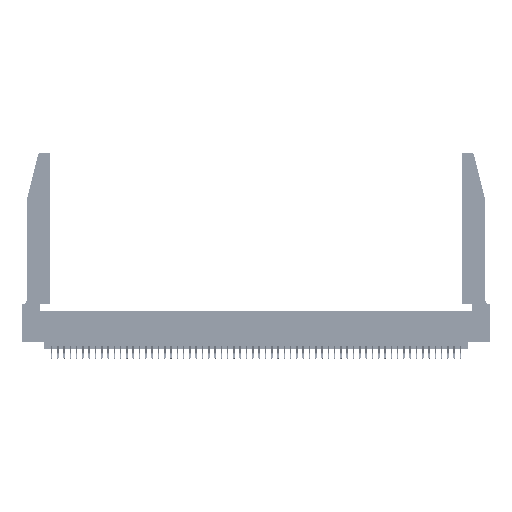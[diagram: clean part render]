
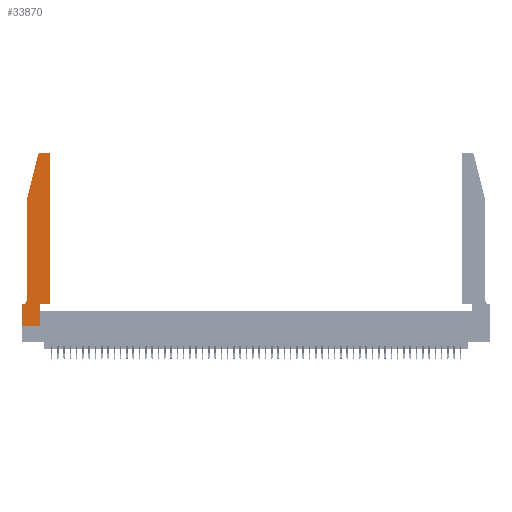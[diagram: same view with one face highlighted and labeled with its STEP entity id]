
A CAD part, top view. The second image highlights one B-rep face of the part: STEP entity #33870.
In plain terms, the highlighted planar face has unit normal (0, 0, 1).
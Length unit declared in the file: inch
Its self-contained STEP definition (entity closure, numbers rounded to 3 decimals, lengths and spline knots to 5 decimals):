
#320 = CARTESIAN_POINT ( 'NONE',  ( 0.0055, 0.35, 0.37 ) ) ;
#573 = LINE ( 'NONE', #35285, #25975 ) ;
#714 = LINE ( 'NONE', #33054, #20214 ) ;
#1095 = DIRECTION ( 'NONE',  ( 1., 0., 0. ) ) ;
#1208 = DIRECTION ( 'NONE',  ( 1., 0., 0. ) ) ;
#1482 = VECTOR ( 'NONE', #1095, 39.37008 ) ;
#1571 = CARTESIAN_POINT ( 'NONE',  ( 0.4205, 2.75, 0.37 ) ) ;
#1722 = VERTEX_POINT ( 'NONE', #13991 ) ;
#2215 = CARTESIAN_POINT ( 'NONE',  ( 0.4505, 2.72, 0.37 ) ) ;
#2318 = CARTESIAN_POINT ( 'NONE',  ( 0.25487, 2.72718, 0.37 ) ) ;
#3125 = CARTESIAN_POINT ( 'NONE',  ( 0.284, 2.75, 0.37 ) ) ;
#3454 = DIRECTION ( 'NONE',  ( -1., 0., 0. ) ) ;
#3720 = DIRECTION ( 'NONE',  ( -1., 0., 0. ) ) ;
#4032 = EDGE_CURVE ( 'NONE', #37979, #1722, #18860, .T. ) ;
#5062 = LINE ( 'NONE', #25738, #34886 ) ;
#6139 = CIRCLE ( 'NONE', #44516, 0.07 ) ;
#6187 = DIRECTION ( 'NONE',  ( 1., 0., 0. ) ) ;
#6192 = VECTOR ( 'NONE', #19793, 39.37008 ) ;
#6794 = FACE_OUTER_BOUND ( 'NONE', #23313, .T. ) ;
#6897 = ORIENTED_EDGE ( 'NONE', *, *, #30292, .T. ) ;
#7027 = ORIENTED_EDGE ( 'NONE', *, *, #11025, .T. ) ;
#8003 = CARTESIAN_POINT ( 'NONE',  ( 0.0055, 0.42, 0.37 ) ) ;
#8296 = DIRECTION ( 'NONE',  ( 1., 0., 0. ) ) ;
#9598 = CARTESIAN_POINT ( 'NONE',  ( 0.284, 2.72, 0.37 ) ) ;
#9760 = ORIENTED_EDGE ( 'NONE', *, *, #29949, .T. ) ;
#9822 = ORIENTED_EDGE ( 'NONE', *, *, #43814, .T. ) ;
#10663 = DIRECTION ( 'NONE',  ( -0.239, -0.971, 0. ) ) ;
#11025 = EDGE_CURVE ( 'NONE', #13094, #11939, #714, .T. ) ;
#11257 = DIRECTION ( 'NONE',  ( 0., -1., 0. ) ) ;
#11314 = LINE ( 'NONE', #20490, #43032 ) ;
#11939 = VERTEX_POINT ( 'NONE', #3125 ) ;
#12610 = CARTESIAN_POINT ( 'NONE',  ( 0.0755, 2., 0.37 ) ) ;
#13094 = VERTEX_POINT ( 'NONE', #1571 ) ;
#13742 = DIRECTION ( 'NONE',  ( 0., 0., 1. ) ) ;
#13981 = DIRECTION ( 'NONE',  ( 0., 0., 1. ) ) ;
#13991 = CARTESIAN_POINT ( 'NONE',  ( 0.4505, 0.35, 0.37 ) ) ;
#15262 = CARTESIAN_POINT ( 'NONE',  ( 0., 0., 0.37 ) ) ;
#15283 = CARTESIAN_POINT ( 'NONE',  ( 0.0755, 2., 0.37 ) ) ;
#16522 = DIRECTION ( 'NONE',  ( 0., 0., -1. ) ) ;
#16576 = VERTEX_POINT ( 'NONE', #320 ) ;
#18341 = PLANE ( 'NONE',  #24719 ) ;
#18860 = LINE ( 'NONE', #29109, #21410 ) ;
#19793 = DIRECTION ( 'NONE',  ( 0., -1., 0. ) ) ;
#19970 = DIRECTION ( 'NONE',  ( 0., 1., 0. ) ) ;
#20214 = VECTOR ( 'NONE', #3720, 39.37008 ) ;
#20245 = DIRECTION ( 'NONE',  ( 0., 0., 1. ) ) ;
#20411 = AXIS2_PLACEMENT_3D ( 'NONE', #9598, #13742, #1208 ) ;
#20490 = CARTESIAN_POINT ( 'NONE',  ( 0.2865, 0.35, 0.37 ) ) ;
#21410 = VECTOR ( 'NONE', #50491, 39.37008 ) ;
#21869 = EDGE_CURVE ( 'NONE', #35267, #13094, #24520, .T. ) ;
#22278 = LINE ( 'NONE', #46572, #1482 ) ;
#22293 = DIRECTION ( 'NONE',  ( 0., 1., 0. ) ) ;
#22319 = CARTESIAN_POINT ( 'NONE',  ( 0., 0.35, 0.37 ) ) ;
#22506 = VECTOR ( 'NONE', #49002, 39.37008 ) ;
#23307 = CARTESIAN_POINT ( 'NONE',  ( 0.0755, 0.35, 0.37 ) ) ;
#23313 = EDGE_LOOP ( 'NONE', ( #7027, #6897, #34327, #27683, #42469, #36609, #9760, #9822, #49058, #27471, #25075, #28129 ) ) ;
#23492 = VERTEX_POINT ( 'NONE', #2318 ) ;
#24485 = EDGE_CURVE ( 'NONE', #45077, #16576, #6139, .T. ) ;
#24520 = CIRCLE ( 'NONE', #27499, 0.03 ) ;
#24719 = AXIS2_PLACEMENT_3D ( 'NONE', #22319, #13981, #6187 ) ;
#25003 = LINE ( 'NONE', #15283, #6192 ) ;
#25075 = ORIENTED_EDGE ( 'NONE', *, *, #37473, .T. ) ;
#25738 = CARTESIAN_POINT ( 'NONE',  ( 0.4505, 0.35, 0.37 ) ) ;
#25975 = VECTOR ( 'NONE', #10663, 39.37008 ) ;
#26600 = VERTEX_POINT ( 'NONE', #12610 ) ;
#27471 = ORIENTED_EDGE ( 'NONE', *, *, #4032, .T. ) ;
#27499 = AXIS2_PLACEMENT_3D ( 'NONE', #49752, #20245, #8296 ) ;
#27683 = ORIENTED_EDGE ( 'NONE', *, *, #31642, .T. ) ;
#28129 = ORIENTED_EDGE ( 'NONE', *, *, #21869, .T. ) ;
#28328 = CIRCLE ( 'NONE', #20411, 0.03 ) ;
#29109 = CARTESIAN_POINT ( 'NONE',  ( 0.4505, 0.35, 0.37 ) ) ;
#29949 = EDGE_CURVE ( 'NONE', #53363, #44378, #47187, .T. ) ;
#30292 = EDGE_CURVE ( 'NONE', #11939, #23492, #28328, .T. ) ;
#31088 = VERTEX_POINT ( 'NONE', #40963 ) ;
#31642 = EDGE_CURVE ( 'NONE', #26600, #45077, #25003, .T. ) ;
#33054 = CARTESIAN_POINT ( 'NONE',  ( 0.2605, 2.75, 0.37 ) ) ;
#33247 = CARTESIAN_POINT ( 'NONE',  ( 0.0755, 0.42, 0.37 ) ) ;
#33271 = CARTESIAN_POINT ( 'NONE',  ( 0.2865, 0.35, 0.37 ) ) ;
#33870 = ADVANCED_FACE ( 'NONE', ( #6794 ), #18341, .T. ) ;
#34189 = VECTOR ( 'NONE', #11257, 39.37008 ) ;
#34327 = ORIENTED_EDGE ( 'NONE', *, *, #36499, .T. ) ;
#34886 = VECTOR ( 'NONE', #22293, 39.37008 ) ;
#35267 = VERTEX_POINT ( 'NONE', #2215 ) ;
#35285 = CARTESIAN_POINT ( 'NONE',  ( 0.0755, 2., 0.37 ) ) ;
#36499 = EDGE_CURVE ( 'NONE', #23492, #26600, #573, .T. ) ;
#36609 = ORIENTED_EDGE ( 'NONE', *, *, #38343, .T. ) ;
#37473 = EDGE_CURVE ( 'NONE', #1722, #35267, #5062, .T. ) ;
#37979 = VERTEX_POINT ( 'NONE', #33271 ) ;
#38343 = EDGE_CURVE ( 'NONE', #16576, #53363, #43822, .T. ) ;
#40963 = CARTESIAN_POINT ( 'NONE',  ( 0.2865, 0., 0.37 ) ) ;
#42469 = ORIENTED_EDGE ( 'NONE', *, *, #24485, .T. ) ;
#43032 = VECTOR ( 'NONE', #19970, 39.37008 ) ;
#43814 = EDGE_CURVE ( 'NONE', #44378, #31088, #22278, .T. ) ;
#43822 = LINE ( 'NONE', #23307, #22506 ) ;
#44378 = VERTEX_POINT ( 'NONE', #49614 ) ;
#44516 = AXIS2_PLACEMENT_3D ( 'NONE', #8003, #16522, #3454 ) ;
#45077 = VERTEX_POINT ( 'NONE', #33247 ) ;
#46572 = CARTESIAN_POINT ( 'NONE',  ( 0., 0., 0.37 ) ) ;
#47187 = LINE ( 'NONE', #15262, #34189 ) ;
#49002 = DIRECTION ( 'NONE',  ( -1., 0., 0. ) ) ;
#49058 = ORIENTED_EDGE ( 'NONE', *, *, #50431, .T. ) ;
#49614 = CARTESIAN_POINT ( 'NONE',  ( 0., 0., 0.37 ) ) ;
#49752 = CARTESIAN_POINT ( 'NONE',  ( 0.4205, 2.72, 0.37 ) ) ;
#50431 = EDGE_CURVE ( 'NONE', #31088, #37979, #11314, .T. ) ;
#50491 = DIRECTION ( 'NONE',  ( 1., 0., 0. ) ) ;
#52891 = CARTESIAN_POINT ( 'NONE',  ( 0., 0.35, 0.37 ) ) ;
#53363 = VERTEX_POINT ( 'NONE', #52891 ) ;
